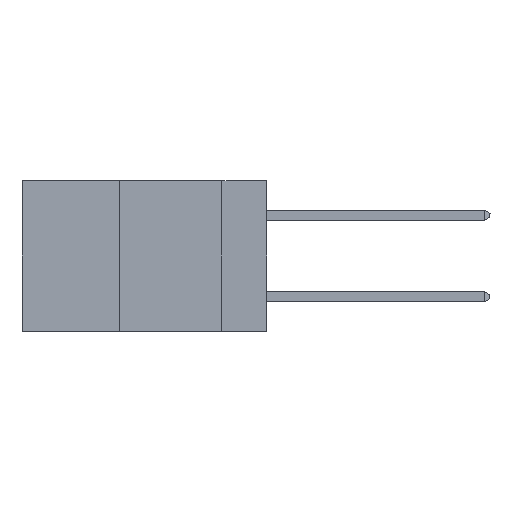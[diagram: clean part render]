
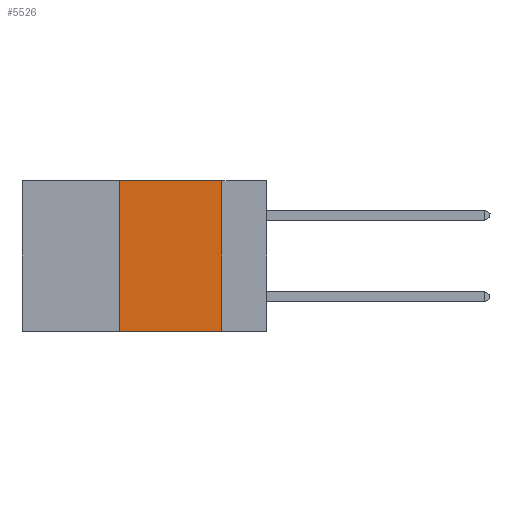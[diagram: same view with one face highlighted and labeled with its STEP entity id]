
A CAD part, left-side view. The second image highlights one B-rep face of the part: STEP entity #5526.
In plain terms, the highlighted planar face has unit normal (-1, 0, 0).
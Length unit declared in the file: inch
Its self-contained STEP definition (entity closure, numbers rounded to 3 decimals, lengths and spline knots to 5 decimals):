
#374 = EDGE_CURVE ( 'NONE', #3082, #8393, #11510, .T. ) ;
#1017 = VECTOR ( 'NONE', #9347, 39.37008 ) ;
#1094 = ORIENTED_EDGE ( 'NONE', *, *, #374, .F. ) ;
#1348 = CARTESIAN_POINT ( 'NONE',  ( 0., 0.36, 0. ) ) ;
#3082 = VERTEX_POINT ( 'NONE', #12316 ) ;
#3392 = DIRECTION ( 'NONE',  ( 0., 0., -1. ) ) ;
#5526 = ADVANCED_FACE ( 'NONE', ( #9760 ), #15856, .F. ) ;
#6002 = DIRECTION ( 'NONE',  ( 1., 0., 0. ) ) ;
#6048 = LINE ( 'NONE', #13836, #25457 ) ;
#8114 = DIRECTION ( 'NONE',  ( 0., 0., -1. ) ) ;
#8393 = VERTEX_POINT ( 'NONE', #20583 ) ;
#9347 = DIRECTION ( 'NONE',  ( 0., -1., 0. ) ) ;
#9760 = FACE_OUTER_BOUND ( 'NONE', #17693, .T. ) ;
#11177 = LINE ( 'NONE', #21425, #1017 ) ;
#11510 = LINE ( 'NONE', #13465, #23831 ) ;
#12316 = CARTESIAN_POINT ( 'NONE',  ( 0., 0.36, 0. ) ) ;
#13022 = VERTEX_POINT ( 'NONE', #17481 ) ;
#13073 = DIRECTION ( 'NONE',  ( 0., 0., 1. ) ) ;
#13202 = ORIENTED_EDGE ( 'NONE', *, *, #22908, .T. ) ;
#13465 = CARTESIAN_POINT ( 'NONE',  ( 0., 0.6, 0. ) ) ;
#13836 = CARTESIAN_POINT ( 'NONE',  ( 0., 0.11, 0. ) ) ;
#14902 = VECTOR ( 'NONE', #13073, 39.37008 ) ;
#15856 = PLANE ( 'NONE',  #24060 ) ;
#15997 = LINE ( 'NONE', #1348, #14902 ) ;
#17047 = EDGE_CURVE ( 'NONE', #17664, #3082, #15997, .T. ) ;
#17481 = CARTESIAN_POINT ( 'NONE',  ( 0., 0.11, -0.37 ) ) ;
#17664 = VERTEX_POINT ( 'NONE', #21022 ) ;
#17693 = EDGE_LOOP ( 'NONE', ( #20267, #1094, #23187, #13202 ) ) ;
#18427 = EDGE_CURVE ( 'NONE', #8393, #13022, #6048, .T. ) ;
#19675 = DIRECTION ( 'NONE',  ( 0., -1., 0. ) ) ;
#20267 = ORIENTED_EDGE ( 'NONE', *, *, #18427, .F. ) ;
#20583 = CARTESIAN_POINT ( 'NONE',  ( 0., 0.11, 0. ) ) ;
#21022 = CARTESIAN_POINT ( 'NONE',  ( 0., 0.36, -0.37 ) ) ;
#21425 = CARTESIAN_POINT ( 'NONE',  ( 0., 0.6, -0.37 ) ) ;
#22908 = EDGE_CURVE ( 'NONE', #17664, #13022, #11177, .T. ) ;
#23187 = ORIENTED_EDGE ( 'NONE', *, *, #17047, .F. ) ;
#23831 = VECTOR ( 'NONE', #19675, 39.37008 ) ;
#23832 = CARTESIAN_POINT ( 'NONE',  ( 0., 0.6, 0. ) ) ;
#24060 = AXIS2_PLACEMENT_3D ( 'NONE', #23832, #6002, #3392 ) ;
#25457 = VECTOR ( 'NONE', #8114, 39.37008 ) ;
